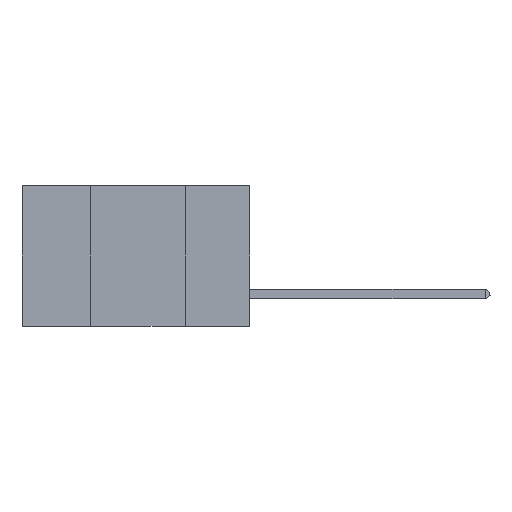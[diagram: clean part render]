
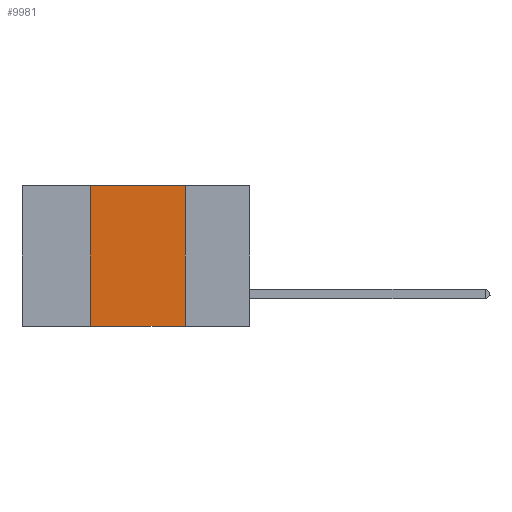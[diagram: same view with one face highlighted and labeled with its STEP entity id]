
A CAD part, left-side view. The second image highlights one B-rep face of the part: STEP entity #9981.
In plain terms, the highlighted planar face has unit normal (-1, 0, 0).
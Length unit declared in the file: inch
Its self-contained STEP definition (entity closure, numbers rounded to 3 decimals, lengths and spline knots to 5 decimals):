
#252 = EDGE_CURVE ( 'NONE', #1753, #7844, #1873, .T. ) ;
#592 = CARTESIAN_POINT ( 'NONE',  ( 0., 0.42, 0. ) ) ;
#1161 = EDGE_LOOP ( 'NONE', ( #5118, #3166, #4121, #10318 ) ) ;
#1753 = VERTEX_POINT ( 'NONE', #3534 ) ;
#1873 = LINE ( 'NONE', #9196, #12405 ) ;
#2316 = PLANE ( 'NONE',  #4515 ) ;
#3166 = ORIENTED_EDGE ( 'NONE', *, *, #6159, .F. ) ;
#3412 = DIRECTION ( 'NONE',  ( 0., -1., 0. ) ) ;
#3534 = CARTESIAN_POINT ( 'NONE',  ( 0., 0.42, -0.37 ) ) ;
#4121 = ORIENTED_EDGE ( 'NONE', *, *, #252, .F. ) ;
#4289 = CARTESIAN_POINT ( 'NONE',  ( 0., 0.17, 0. ) ) ;
#4515 = AXIS2_PLACEMENT_3D ( 'NONE', #7121, #11830, #4795 ) ;
#4526 = CARTESIAN_POINT ( 'NONE',  ( 0., 0.6, 0. ) ) ;
#4795 = DIRECTION ( 'NONE',  ( 0., 0., -1. ) ) ;
#5091 = VECTOR ( 'NONE', #3412, 39.37008 ) ;
#5118 = ORIENTED_EDGE ( 'NONE', *, *, #9695, .F. ) ;
#5730 = VERTEX_POINT ( 'NONE', #14584 ) ;
#6159 = EDGE_CURVE ( 'NONE', #7844, #12684, #13187, .T. ) ;
#6593 = DIRECTION ( 'NONE',  ( 0., 0., -1. ) ) ;
#7121 = CARTESIAN_POINT ( 'NONE',  ( 0., 0.6, 0. ) ) ;
#7844 = VERTEX_POINT ( 'NONE', #592 ) ;
#9196 = CARTESIAN_POINT ( 'NONE',  ( 0., 0.42, 0. ) ) ;
#9695 = EDGE_CURVE ( 'NONE', #12684, #5730, #10877, .T. ) ;
#9981 = ADVANCED_FACE ( 'NONE', ( #13049 ), #2316, .F. ) ;
#9988 = CARTESIAN_POINT ( 'NONE',  ( 0., 0.17, 0. ) ) ;
#10318 = ORIENTED_EDGE ( 'NONE', *, *, #14791, .T. ) ;
#10877 = LINE ( 'NONE', #4289, #11605 ) ;
#11605 = VECTOR ( 'NONE', #6593, 39.37008 ) ;
#11614 = DIRECTION ( 'NONE',  ( 0., 0., 1. ) ) ;
#11830 = DIRECTION ( 'NONE',  ( 1., 0., 0. ) ) ;
#12405 = VECTOR ( 'NONE', #11614, 39.37008 ) ;
#12684 = VERTEX_POINT ( 'NONE', #9988 ) ;
#13049 = FACE_OUTER_BOUND ( 'NONE', #1161, .T. ) ;
#13187 = LINE ( 'NONE', #4526, #15029 ) ;
#13439 = LINE ( 'NONE', #15090, #5091 ) ;
#14584 = CARTESIAN_POINT ( 'NONE',  ( 0., 0.17, -0.37 ) ) ;
#14781 = DIRECTION ( 'NONE',  ( 0., -1., 0. ) ) ;
#14791 = EDGE_CURVE ( 'NONE', #1753, #5730, #13439, .T. ) ;
#15029 = VECTOR ( 'NONE', #14781, 39.37008 ) ;
#15090 = CARTESIAN_POINT ( 'NONE',  ( 0., 0.6, -0.37 ) ) ;
